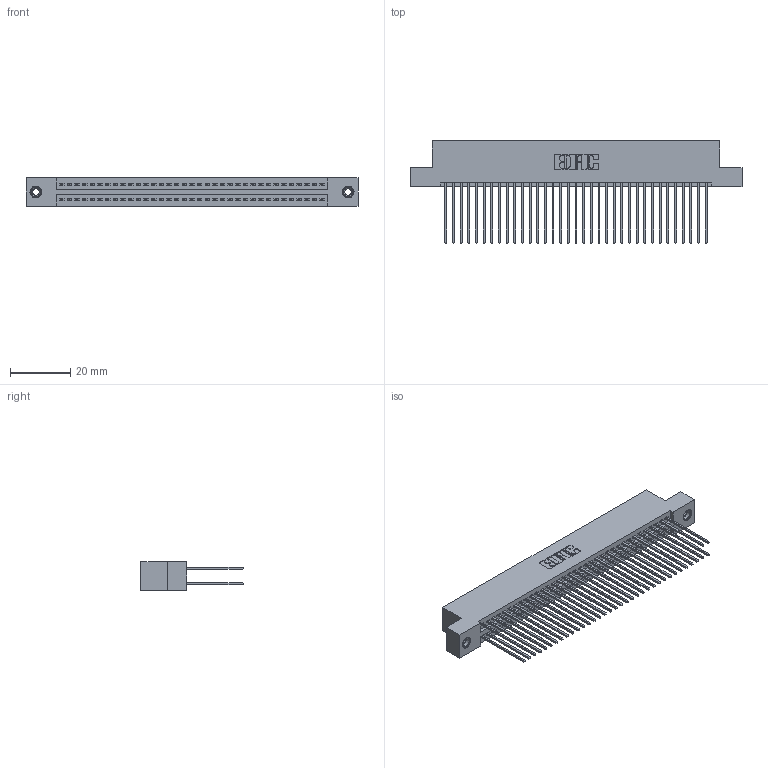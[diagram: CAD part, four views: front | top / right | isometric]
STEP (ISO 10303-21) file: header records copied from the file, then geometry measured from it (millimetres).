
FILE_DESCRIPTION (( 'STEP AP203' ), '1' );
FILE_NAME ('395-070-541-208.STEP', '2019-10-24T01:01:38', ( '' ), ( '' ), 'SwSTEP 2.0', 'SolidWorks 2016', '' );
FILE_SCHEMA (( 'CONFIG_CONTROL_DESIGN' ));
Length unit declared in the file: inch
Products named in the file (4): 345 Part_Flush Mounting Lugs - 0.156 Dia-TI; 345-292-001_345-293-141; 345-250-001_345-250-003-102; 395-070-541-208
Assembly tree (73 placements, depth 2):
  395-070-541-208
    345 Part_Flush Mounting Lugs - 0.156 Dia-TI
    345-292-001_345-293-141  x70
    345-250-001_345-250-003-102  x2
Bounding box: 110.11 x 33.96 x 9.4 mm (x, y, z)
Volume: 11026.2 mm3; surface area: 18064.3 mm2
Topology: 73 solids, 73 shells, 3686 faces, 10907 edges, 7170 vertices
Faces by surface type: plane 2422, cylinder 1248, cone 12, torus 4
Entity records: 29608 total; most frequent: CARTESIAN_POINT 4951, ORIENTED_EDGE 4878, DIRECTION 4401, EDGE_CURVE 2439, VECTOR 2147, LINE 2147, VERTEX_POINT 1620, AXIS2_PLACEMENT_3D 1127
